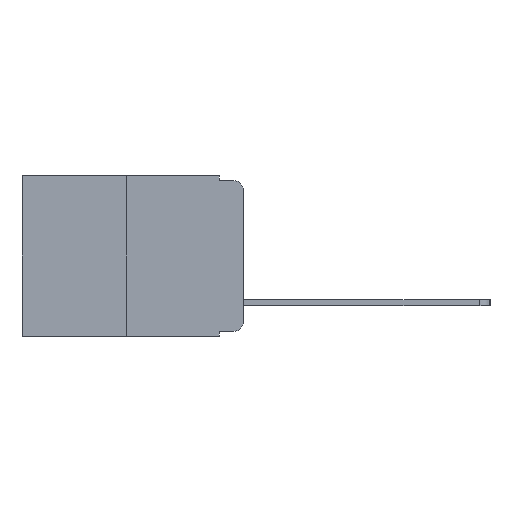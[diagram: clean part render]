
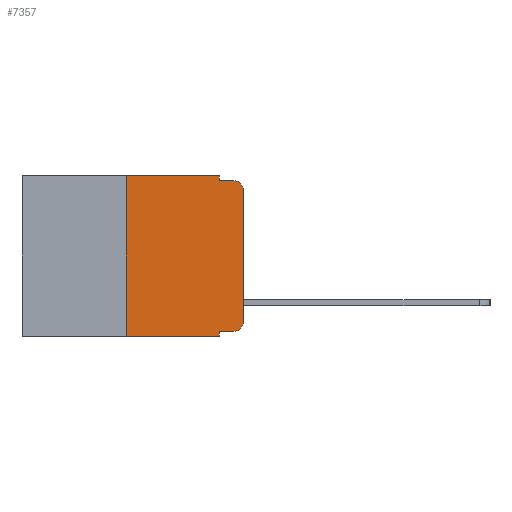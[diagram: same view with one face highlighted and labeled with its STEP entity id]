
A CAD part, left-side view. The second image highlights one B-rep face of the part: STEP entity #7357.
In plain terms, the highlighted planar face has unit normal (-1, 0, 0).
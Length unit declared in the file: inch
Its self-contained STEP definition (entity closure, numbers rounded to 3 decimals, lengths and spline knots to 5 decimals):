
#12 = CARTESIAN_POINT ( 'NONE',  ( 0., 0.051, 0. ) ) ;
#185 = ORIENTED_EDGE ( 'NONE', *, *, #12014, .F. ) ;
#213 = CIRCLE ( 'NONE', #274, 0.02 ) ;
#274 = AXIS2_PLACEMENT_3D ( 'NONE', #6851, #468, #7926 ) ;
#284 = LINE ( 'NONE', #9238, #11471 ) ;
#392 = DIRECTION ( 'NONE',  ( 1., 0., 0. ) ) ;
#468 = DIRECTION ( 'NONE',  ( -1., 0., 0. ) ) ;
#525 = CARTESIAN_POINT ( 'NONE',  ( 0., 0.051, 0. ) ) ;
#1152 = ORIENTED_EDGE ( 'NONE', *, *, #11595, .T. ) ;
#1429 = VECTOR ( 'NONE', #9163, 39.37008 ) ;
#2295 = CARTESIAN_POINT ( 'NONE',  ( 0., 0.473, 0. ) ) ;
#2490 = EDGE_CURVE ( 'NONE', #7371, #6459, #12503, .T. ) ;
#3048 = EDGE_CURVE ( 'NONE', #11600, #7371, #9074, .T. ) ;
#3060 = DIRECTION ( 'NONE',  ( -1., 0., 0. ) ) ;
#3069 = CARTESIAN_POINT ( 'NONE',  ( 0., 0.25, 0. ) ) ;
#3366 = DIRECTION ( 'NONE',  ( 0., 0., 1. ) ) ;
#3387 = ORIENTED_EDGE ( 'NONE', *, *, #3048, .F. ) ;
#4048 = VECTOR ( 'NONE', #11512, 39.37008 ) ;
#4201 = CARTESIAN_POINT ( 'NONE',  ( 0., 0.051, -0.333 ) ) ;
#4366 = DIRECTION ( 'NONE',  ( 0., -1., 0. ) ) ;
#4430 = VECTOR ( 'NONE', #3366, 39.37008 ) ;
#4669 = CARTESIAN_POINT ( 'NONE',  ( 0., 0.051, -0.01 ) ) ;
#4772 = LINE ( 'NONE', #5451, #4430 ) ;
#5197 = ORIENTED_EDGE ( 'NONE', *, *, #2490, .F. ) ;
#5262 = EDGE_CURVE ( 'NONE', #8803, #6251, #6534, .T. ) ;
#5451 = CARTESIAN_POINT ( 'NONE',  ( 0., 0., 0. ) ) ;
#5467 = CARTESIAN_POINT ( 'NONE',  ( 0., 0.051, -0.333 ) ) ;
#5476 = VERTEX_POINT ( 'NONE', #13012 ) ;
#5704 = LINE ( 'NONE', #2295, #10920 ) ;
#5775 = CARTESIAN_POINT ( 'NONE',  ( 0., 0.051, 0. ) ) ;
#5860 = ORIENTED_EDGE ( 'NONE', *, *, #5262, .T. ) ;
#5883 = EDGE_CURVE ( 'NONE', #10097, #11600, #5704, .T. ) ;
#5886 = VECTOR ( 'NONE', #10643, 39.37008 ) ;
#6129 = VERTEX_POINT ( 'NONE', #9018 ) ;
#6251 = VERTEX_POINT ( 'NONE', #8214 ) ;
#6459 = VERTEX_POINT ( 'NONE', #10599 ) ;
#6534 = LINE ( 'NONE', #4201, #4048 ) ;
#6764 = CARTESIAN_POINT ( 'NONE',  ( 0., 0.473, 0. ) ) ;
#6823 = AXIS2_PLACEMENT_3D ( 'NONE', #9421, #3060, #10441 ) ;
#6851 = CARTESIAN_POINT ( 'NONE',  ( 0., 0.02, -0.313 ) ) ;
#7124 = AXIS2_PLACEMENT_3D ( 'NONE', #6764, #392, #7861 ) ;
#7357 = ADVANCED_FACE ( 'NONE', ( #9182 ), #7810, .F. ) ;
#7371 = VERTEX_POINT ( 'NONE', #4669 ) ;
#7580 = VECTOR ( 'NONE', #4366, 39.37008 ) ;
#7709 = ORIENTED_EDGE ( 'NONE', *, *, #13153, .T. ) ;
#7810 = PLANE ( 'NONE',  #7124 ) ;
#7861 = DIRECTION ( 'NONE',  ( 0., 0., -1. ) ) ;
#7926 = DIRECTION ( 'NONE',  ( 0., 0., -1. ) ) ;
#7970 = DIRECTION ( 'NONE',  ( 0., 0., -1. ) ) ;
#8214 = CARTESIAN_POINT ( 'NONE',  ( 0., 0.02, -0.333 ) ) ;
#8637 = EDGE_LOOP ( 'NONE', ( #12467, #7709, #5197, #3387, #12315, #10326, #12173, #185, #5860, #1152 ) ) ;
#8725 = VECTOR ( 'NONE', #7970, 39.37008 ) ;
#8734 = LINE ( 'NONE', #12, #5886 ) ;
#8803 = VERTEX_POINT ( 'NONE', #5467 ) ;
#9018 = CARTESIAN_POINT ( 'NONE',  ( 0., 0., -0.03 ) ) ;
#9074 = LINE ( 'NONE', #525, #8725 ) ;
#9163 = DIRECTION ( 'NONE',  ( 0., -1., 0. ) ) ;
#9182 = FACE_OUTER_BOUND ( 'NONE', #8637, .T. ) ;
#9195 = EDGE_CURVE ( 'NONE', #10559, #10097, #284, .T. ) ;
#9238 = CARTESIAN_POINT ( 'NONE',  ( 0., 0.25, 0. ) ) ;
#9421 = CARTESIAN_POINT ( 'NONE',  ( 0., 0.02, -0.03 ) ) ;
#9422 = CARTESIAN_POINT ( 'NONE',  ( 0., 0.25, -0.343 ) ) ;
#9540 = EDGE_CURVE ( 'NONE', #5476, #6129, #4772, .T. ) ;
#9729 = DIRECTION ( 'NONE',  ( 0., -1., 0. ) ) ;
#9794 = VERTEX_POINT ( 'NONE', #10986 ) ;
#10097 = VERTEX_POINT ( 'NONE', #3069 ) ;
#10326 = ORIENTED_EDGE ( 'NONE', *, *, #9195, .F. ) ;
#10441 = DIRECTION ( 'NONE',  ( 0., 0., -1. ) ) ;
#10559 = VERTEX_POINT ( 'NONE', #9422 ) ;
#10599 = CARTESIAN_POINT ( 'NONE',  ( 0., 0.02, -0.01 ) ) ;
#10643 = DIRECTION ( 'NONE',  ( 0., 0., -1. ) ) ;
#10920 = VECTOR ( 'NONE', #9729, 39.37008 ) ;
#10986 = CARTESIAN_POINT ( 'NONE',  ( 0., 0.051, -0.343 ) ) ;
#11217 = CIRCLE ( 'NONE', #6823, 0.02 ) ;
#11433 = EDGE_CURVE ( 'NONE', #10559, #9794, #12955, .T. ) ;
#11471 = VECTOR ( 'NONE', #12187, 39.37008 ) ;
#11512 = DIRECTION ( 'NONE',  ( 0., -1., 0. ) ) ;
#11595 = EDGE_CURVE ( 'NONE', #6251, #5476, #213, .T. ) ;
#11600 = VERTEX_POINT ( 'NONE', #5775 ) ;
#12014 = EDGE_CURVE ( 'NONE', #8803, #9794, #8734, .T. ) ;
#12173 = ORIENTED_EDGE ( 'NONE', *, *, #11433, .T. ) ;
#12187 = DIRECTION ( 'NONE',  ( 0., 0., 1. ) ) ;
#12315 = ORIENTED_EDGE ( 'NONE', *, *, #5883, .F. ) ;
#12467 = ORIENTED_EDGE ( 'NONE', *, *, #9540, .T. ) ;
#12503 = LINE ( 'NONE', #13096, #1429 ) ;
#12692 = CARTESIAN_POINT ( 'NONE',  ( 0., 0.473, -0.343 ) ) ;
#12955 = LINE ( 'NONE', #12692, #7580 ) ;
#13012 = CARTESIAN_POINT ( 'NONE',  ( 0., 0., -0.313 ) ) ;
#13096 = CARTESIAN_POINT ( 'NONE',  ( 0., 0.051, -0.01 ) ) ;
#13153 = EDGE_CURVE ( 'NONE', #6129, #6459, #11217, .T. ) ;
